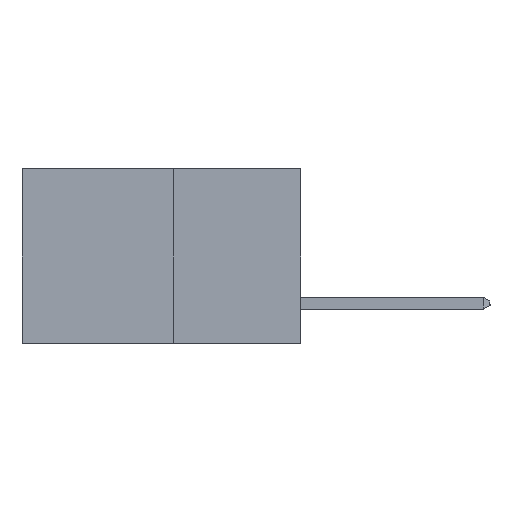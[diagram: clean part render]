
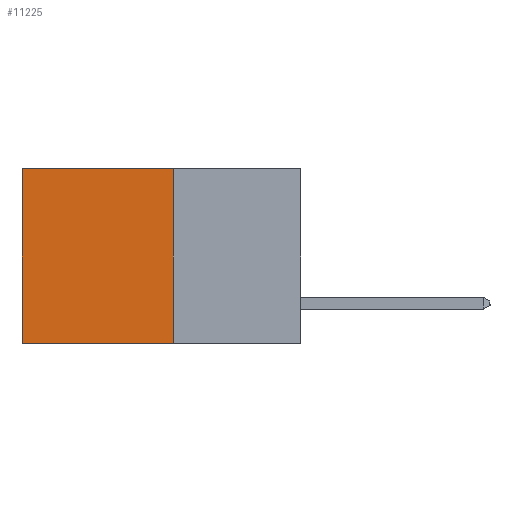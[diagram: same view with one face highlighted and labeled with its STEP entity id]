
A CAD part, left-side view. The second image highlights one B-rep face of the part: STEP entity #11225.
In plain terms, the highlighted planar face has unit normal (-1, 0, 0).
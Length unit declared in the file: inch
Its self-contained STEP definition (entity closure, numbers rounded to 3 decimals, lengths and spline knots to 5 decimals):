
#451 = FACE_OUTER_BOUND ( 'NONE', #13236, .T. ) ;
#588 = EDGE_CURVE ( 'NONE', #3122, #1169, #2709, .T. ) ;
#1169 = VERTEX_POINT ( 'NONE', #13325 ) ;
#1807 = CARTESIAN_POINT ( 'NONE',  ( 0.277, 0.27, -0.37 ) ) ;
#2159 = LINE ( 'NONE', #1807, #12892 ) ;
#2500 = EDGE_CURVE ( 'NONE', #2816, #8849, #12259, .T. ) ;
#2709 = LINE ( 'NONE', #13366, #11332 ) ;
#2816 = VERTEX_POINT ( 'NONE', #6888 ) ;
#3122 = VERTEX_POINT ( 'NONE', #13532 ) ;
#3541 = ORIENTED_EDGE ( 'NONE', *, *, #7988, .T. ) ;
#3954 = DIRECTION ( 'NONE',  ( 0., 1., 0. ) ) ;
#4367 = CARTESIAN_POINT ( 'NONE',  ( 0.277, 0.27, -0.37 ) ) ;
#5137 = DIRECTION ( 'NONE',  ( 0., 0., -1. ) ) ;
#5369 = CARTESIAN_POINT ( 'NONE',  ( 0.277, 0.27, 0. ) ) ;
#5397 = DIRECTION ( 'NONE',  ( 0., 0., -1. ) ) ;
#5782 = ORIENTED_EDGE ( 'NONE', *, *, #588, .F. ) ;
#6888 = CARTESIAN_POINT ( 'NONE',  ( 0.277, 0.59, 0. ) ) ;
#7056 = CARTESIAN_POINT ( 'NONE',  ( 0.277, 0.59, -0.37 ) ) ;
#7988 = EDGE_CURVE ( 'NONE', #3122, #2816, #11289, .T. ) ;
#8277 = EDGE_CURVE ( 'NONE', #1169, #8849, #2159, .T. ) ;
#8832 = VECTOR ( 'NONE', #11588, 39.37008 ) ;
#8849 = VERTEX_POINT ( 'NONE', #7056 ) ;
#8859 = AXIS2_PLACEMENT_3D ( 'NONE', #4367, #11578, #5397 ) ;
#9442 = ORIENTED_EDGE ( 'NONE', *, *, #2500, .T. ) ;
#9493 = VECTOR ( 'NONE', #13275, 39.37008 ) ;
#9962 = ORIENTED_EDGE ( 'NONE', *, *, #8277, .F. ) ;
#10144 = CARTESIAN_POINT ( 'NONE',  ( 0.277, 0.59, -0.37 ) ) ;
#10518 = PLANE ( 'NONE',  #8859 ) ;
#11225 = ADVANCED_FACE ( 'NONE', ( #451 ), #10518, .F. ) ;
#11289 = LINE ( 'NONE', #5369, #8832 ) ;
#11332 = VECTOR ( 'NONE', #5137, 39.37008 ) ;
#11578 = DIRECTION ( 'NONE',  ( 1., 0., 0. ) ) ;
#11588 = DIRECTION ( 'NONE',  ( 0., 1., 0. ) ) ;
#12259 = LINE ( 'NONE', #10144, #9493 ) ;
#12892 = VECTOR ( 'NONE', #3954, 39.37008 ) ;
#13236 = EDGE_LOOP ( 'NONE', ( #9442, #9962, #5782, #3541 ) ) ;
#13275 = DIRECTION ( 'NONE',  ( 0., 0., -1. ) ) ;
#13325 = CARTESIAN_POINT ( 'NONE',  ( 0.277, 0.27, -0.37 ) ) ;
#13366 = CARTESIAN_POINT ( 'NONE',  ( 0.277, 0.27, -0.37 ) ) ;
#13532 = CARTESIAN_POINT ( 'NONE',  ( 0.277, 0.27, 0. ) ) ;
